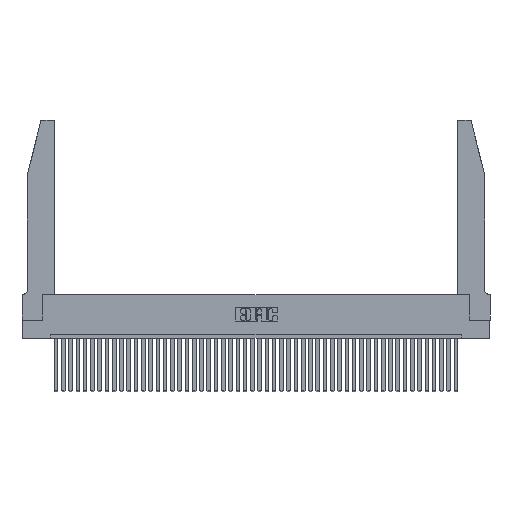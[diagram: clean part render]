
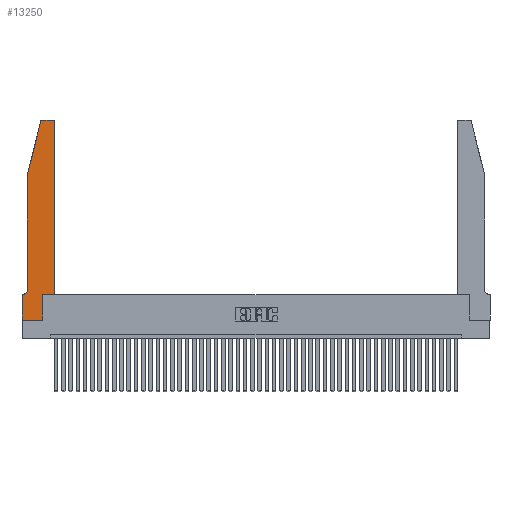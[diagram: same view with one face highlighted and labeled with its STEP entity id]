
A CAD part, top view. The second image highlights one B-rep face of the part: STEP entity #13250.
In plain terms, the highlighted planar face has unit normal (0, 0, 1).
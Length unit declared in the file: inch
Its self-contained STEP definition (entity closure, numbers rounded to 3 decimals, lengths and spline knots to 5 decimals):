
#20 = CIRCLE ( 'NONE', #18279, 0.07 ) ;
#1247 = VECTOR ( 'NONE', #19968, 39.37008 ) ;
#1692 = EDGE_CURVE ( 'NONE', #26175, #18919, #9297, .T. ) ;
#2199 = EDGE_CURVE ( 'NONE', #18919, #13731, #37444, .T. ) ;
#2894 = EDGE_CURVE ( 'NONE', #7750, #10413, #20, .T. ) ;
#2989 = VERTEX_POINT ( 'NONE', #32271 ) ;
#3155 = EDGE_CURVE ( 'NONE', #2989, #15673, #27154, .T. ) ;
#3901 = EDGE_CURVE ( 'NONE', #10413, #37649, #20506, .T. ) ;
#4486 = CARTESIAN_POINT ( 'NONE',  ( 0.4505, 0.35, 0.37 ) ) ;
#4855 = CARTESIAN_POINT ( 'NONE',  ( 0.2605, 2.75, 0.37 ) ) ;
#5129 = FACE_OUTER_BOUND ( 'NONE', #6761, .T. ) ;
#5505 = VECTOR ( 'NONE', #21834, 39.37008 ) ;
#6232 = VECTOR ( 'NONE', #30418, 39.37008 ) ;
#6314 = DIRECTION ( 'NONE',  ( -1., 0., 0. ) ) ;
#6761 = EDGE_LOOP ( 'NONE', ( #19680, #9323, #42571, #33923, #12929, #36529, #8664, #25405, #39871, #31515, #18190, #22522 ) ) ;
#7081 = DIRECTION ( 'NONE',  ( 0., 0., 1. ) ) ;
#7210 = EDGE_CURVE ( 'NONE', #37649, #18470, #26728, .T. ) ;
#7275 = DIRECTION ( 'NONE',  ( 0., 0., -1. ) ) ;
#7750 = VERTEX_POINT ( 'NONE', #17984 ) ;
#8664 = ORIENTED_EDGE ( 'NONE', *, *, #7210, .T. ) ;
#8875 = CARTESIAN_POINT ( 'NONE',  ( 0.25487, 2.72718, 0.37 ) ) ;
#9297 = CIRCLE ( 'NONE', #29364, 0.03 ) ;
#9323 = ORIENTED_EDGE ( 'NONE', *, *, #1692, .T. ) ;
#9645 = DIRECTION ( 'NONE',  ( 1., 0., 0. ) ) ;
#10413 = VERTEX_POINT ( 'NONE', #32818 ) ;
#10421 = CARTESIAN_POINT ( 'NONE',  ( 0., 0.35, 0.37 ) ) ;
#10747 = CARTESIAN_POINT ( 'NONE',  ( 0.4205, 2.75, 0.37 ) ) ;
#11688 = LINE ( 'NONE', #26587, #23680 ) ;
#12251 = EDGE_CURVE ( 'NONE', #27475, #20177, #11688, .T. ) ;
#12929 = ORIENTED_EDGE ( 'NONE', *, *, #2894, .T. ) ;
#13235 = EDGE_CURVE ( 'NONE', #42549, #2989, #21897, .T. ) ;
#13236 = CARTESIAN_POINT ( 'NONE',  ( 0.0755, 0.35, 0.37 ) ) ;
#13250 = ADVANCED_FACE ( 'NONE', ( #5129 ), #40131, .T. ) ;
#13731 = VERTEX_POINT ( 'NONE', #17082 ) ;
#13881 = LINE ( 'NONE', #4855, #16600 ) ;
#14319 = EDGE_CURVE ( 'NONE', #13731, #7750, #19702, .T. ) ;
#14765 = CARTESIAN_POINT ( 'NONE',  ( 0.0755, 2., 0.37 ) ) ;
#15673 = VERTEX_POINT ( 'NONE', #10747 ) ;
#16249 = EDGE_CURVE ( 'NONE', #18470, #27475, #35208, .T. ) ;
#16600 = VECTOR ( 'NONE', #36169, 39.37008 ) ;
#16740 = EDGE_CURVE ( 'NONE', #20177, #42549, #39469, .T. ) ;
#16806 = CARTESIAN_POINT ( 'NONE',  ( 0.2865, 0., 0.37 ) ) ;
#17082 = CARTESIAN_POINT ( 'NONE',  ( 0.0755, 2., 0.37 ) ) ;
#17450 = EDGE_CURVE ( 'NONE', #15673, #26175, #13881, .T. ) ;
#17984 = CARTESIAN_POINT ( 'NONE',  ( 0.0755, 0.42, 0.37 ) ) ;
#18190 = ORIENTED_EDGE ( 'NONE', *, *, #13235, .T. ) ;
#18279 = AXIS2_PLACEMENT_3D ( 'NONE', #24012, #7275, #41614 ) ;
#18470 = VERTEX_POINT ( 'NONE', #32841 ) ;
#18919 = VERTEX_POINT ( 'NONE', #8875 ) ;
#19390 = CARTESIAN_POINT ( 'NONE',  ( 0., 0.35, 0.37 ) ) ;
#19680 = ORIENTED_EDGE ( 'NONE', *, *, #17450, .T. ) ;
#19702 = LINE ( 'NONE', #14765, #1247 ) ;
#19952 = CARTESIAN_POINT ( 'NONE',  ( 0.4505, 0.35, 0.37 ) ) ;
#19968 = DIRECTION ( 'NONE',  ( 0., -1., 0. ) ) ;
#20177 = VERTEX_POINT ( 'NONE', #36852 ) ;
#20506 = LINE ( 'NONE', #13236, #24309 ) ;
#21834 = DIRECTION ( 'NONE',  ( -0.239, -0.971, 0. ) ) ;
#21897 = LINE ( 'NONE', #19952, #6232 ) ;
#22522 = ORIENTED_EDGE ( 'NONE', *, *, #3155, .T. ) ;
#23680 = VECTOR ( 'NONE', #33527, 39.37008 ) ;
#24012 = CARTESIAN_POINT ( 'NONE',  ( 0.0055, 0.42, 0.37 ) ) ;
#24309 = VECTOR ( 'NONE', #6314, 39.37008 ) ;
#24443 = AXIS2_PLACEMENT_3D ( 'NONE', #36329, #7081, #38289 ) ;
#25405 = ORIENTED_EDGE ( 'NONE', *, *, #16249, .T. ) ;
#26175 = VERTEX_POINT ( 'NONE', #42050 ) ;
#26289 = DIRECTION ( 'NONE',  ( 1., 0., 0. ) ) ;
#26587 = CARTESIAN_POINT ( 'NONE',  ( 0.2865, 0.35, 0.37 ) ) ;
#26728 = LINE ( 'NONE', #30217, #40228 ) ;
#27154 = CIRCLE ( 'NONE', #24443, 0.03 ) ;
#27475 = VERTEX_POINT ( 'NONE', #16806 ) ;
#28721 = DIRECTION ( 'NONE',  ( 1., 0., 0. ) ) ;
#29322 = CARTESIAN_POINT ( 'NONE',  ( 0.284, 2.72, 0.37 ) ) ;
#29364 = AXIS2_PLACEMENT_3D ( 'NONE', #29322, #29631, #37162 ) ;
#29631 = DIRECTION ( 'NONE',  ( 0., 0., 1. ) ) ;
#30217 = CARTESIAN_POINT ( 'NONE',  ( 0., 0., 0.37 ) ) ;
#30418 = DIRECTION ( 'NONE',  ( 0., 1., 0. ) ) ;
#30716 = AXIS2_PLACEMENT_3D ( 'NONE', #19390, #35846, #9645 ) ;
#31207 = CARTESIAN_POINT ( 'NONE',  ( 0.4505, 0.35, 0.37 ) ) ;
#31515 = ORIENTED_EDGE ( 'NONE', *, *, #16740, .T. ) ;
#32271 = CARTESIAN_POINT ( 'NONE',  ( 0.4505, 2.72, 0.37 ) ) ;
#32818 = CARTESIAN_POINT ( 'NONE',  ( 0.0055, 0.35, 0.37 ) ) ;
#32841 = CARTESIAN_POINT ( 'NONE',  ( 0., 0., 0.37 ) ) ;
#33527 = DIRECTION ( 'NONE',  ( 0., 1., 0. ) ) ;
#33923 = ORIENTED_EDGE ( 'NONE', *, *, #14319, .T. ) ;
#35208 = LINE ( 'NONE', #42413, #44413 ) ;
#35846 = DIRECTION ( 'NONE',  ( 0., 0., 1. ) ) ;
#36169 = DIRECTION ( 'NONE',  ( -1., 0., 0. ) ) ;
#36329 = CARTESIAN_POINT ( 'NONE',  ( 0.4205, 2.72, 0.37 ) ) ;
#36529 = ORIENTED_EDGE ( 'NONE', *, *, #3901, .T. ) ;
#36852 = CARTESIAN_POINT ( 'NONE',  ( 0.2865, 0.35, 0.37 ) ) ;
#37162 = DIRECTION ( 'NONE',  ( 1., 0., 0. ) ) ;
#37444 = LINE ( 'NONE', #38027, #5505 ) ;
#37649 = VERTEX_POINT ( 'NONE', #10421 ) ;
#38027 = CARTESIAN_POINT ( 'NONE',  ( 0.0755, 2., 0.37 ) ) ;
#38289 = DIRECTION ( 'NONE',  ( 1., 0., 0. ) ) ;
#38354 = VECTOR ( 'NONE', #28721, 39.37008 ) ;
#39469 = LINE ( 'NONE', #4486, #38354 ) ;
#39871 = ORIENTED_EDGE ( 'NONE', *, *, #12251, .T. ) ;
#40018 = DIRECTION ( 'NONE',  ( 0., -1., 0. ) ) ;
#40131 = PLANE ( 'NONE',  #30716 ) ;
#40228 = VECTOR ( 'NONE', #40018, 39.37008 ) ;
#41614 = DIRECTION ( 'NONE',  ( -1., 0., 0. ) ) ;
#42050 = CARTESIAN_POINT ( 'NONE',  ( 0.284, 2.75, 0.37 ) ) ;
#42413 = CARTESIAN_POINT ( 'NONE',  ( 0., 0., 0.37 ) ) ;
#42549 = VERTEX_POINT ( 'NONE', #31207 ) ;
#42571 = ORIENTED_EDGE ( 'NONE', *, *, #2199, .T. ) ;
#44413 = VECTOR ( 'NONE', #26289, 39.37008 ) ;
